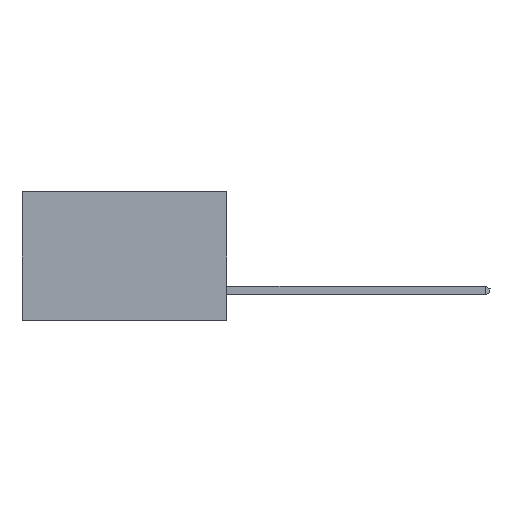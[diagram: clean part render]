
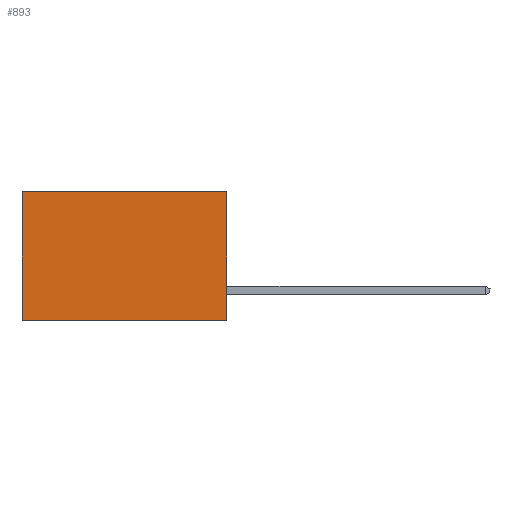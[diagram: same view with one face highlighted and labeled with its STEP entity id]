
A CAD part, left-side view. The second image highlights one B-rep face of the part: STEP entity #893.
In plain terms, the highlighted planar face has unit normal (-1, 0, 0).
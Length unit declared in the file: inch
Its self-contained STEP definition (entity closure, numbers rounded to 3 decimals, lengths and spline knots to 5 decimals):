
#306 = LINE ( 'NONE', #1772, #3655 ) ;
#692 = ORIENTED_EDGE ( 'NONE', *, *, #10455, .T. ) ;
#798 = DIRECTION ( 'NONE',  ( 0., 1., 0. ) ) ;
#893 = ADVANCED_FACE ( 'NONE', ( #13537 ), #10093, .F. ) ;
#1140 = LINE ( 'NONE', #7470, #9564 ) ;
#1278 = EDGE_CURVE ( 'NONE', #12405, #3185, #306, .T. ) ;
#1404 = CARTESIAN_POINT ( 'NONE',  ( 0.277, 0., -0.37 ) ) ;
#1772 = CARTESIAN_POINT ( 'NONE',  ( 0.277, 0., -0.37 ) ) ;
#1819 = DIRECTION ( 'NONE',  ( 0., 0., -1. ) ) ;
#1904 = EDGE_CURVE ( 'NONE', #12405, #6167, #9570, .T. ) ;
#1916 = CARTESIAN_POINT ( 'NONE',  ( 0.277, 0.59, -0.37 ) ) ;
#1956 = DIRECTION ( 'NONE',  ( 0., 1., 0. ) ) ;
#2021 = CARTESIAN_POINT ( 'NONE',  ( 0.277, 0., 0. ) ) ;
#2196 = ORIENTED_EDGE ( 'NONE', *, *, #12901, .F. ) ;
#2802 = DIRECTION ( 'NONE',  ( 0., 0., -1. ) ) ;
#2820 = DIRECTION ( 'NONE',  ( 1., 0., 0. ) ) ;
#3174 = VECTOR ( 'NONE', #1819, 39.37008 ) ;
#3185 = VERTEX_POINT ( 'NONE', #13166 ) ;
#3655 = VECTOR ( 'NONE', #3729, 39.37008 ) ;
#3729 = DIRECTION ( 'NONE',  ( 0., 0., -1. ) ) ;
#4508 = CARTESIAN_POINT ( 'NONE',  ( 0.277, 0.59, -0.37 ) ) ;
#4574 = ORIENTED_EDGE ( 'NONE', *, *, #1278, .F. ) ;
#4985 = ORIENTED_EDGE ( 'NONE', *, *, #1904, .T. ) ;
#5665 = CARTESIAN_POINT ( 'NONE',  ( 0.277, 0.59, 0. ) ) ;
#6167 = VERTEX_POINT ( 'NONE', #5665 ) ;
#6365 = VECTOR ( 'NONE', #798, 39.37008 ) ;
#6436 = LINE ( 'NONE', #1916, #3174 ) ;
#6487 = CARTESIAN_POINT ( 'NONE',  ( 0.277, 0., 0. ) ) ;
#6953 = AXIS2_PLACEMENT_3D ( 'NONE', #1404, #2820, #2802 ) ;
#7470 = CARTESIAN_POINT ( 'NONE',  ( 0.277, 0., -0.37 ) ) ;
#7611 = EDGE_LOOP ( 'NONE', ( #692, #2196, #4574, #4985 ) ) ;
#9564 = VECTOR ( 'NONE', #1956, 39.37008 ) ;
#9570 = LINE ( 'NONE', #6487, #6365 ) ;
#10048 = VERTEX_POINT ( 'NONE', #4508 ) ;
#10093 = PLANE ( 'NONE',  #6953 ) ;
#10455 = EDGE_CURVE ( 'NONE', #6167, #10048, #6436, .T. ) ;
#12405 = VERTEX_POINT ( 'NONE', #2021 ) ;
#12901 = EDGE_CURVE ( 'NONE', #3185, #10048, #1140, .T. ) ;
#13166 = CARTESIAN_POINT ( 'NONE',  ( 0.277, 0., -0.37 ) ) ;
#13537 = FACE_OUTER_BOUND ( 'NONE', #7611, .T. ) ;
